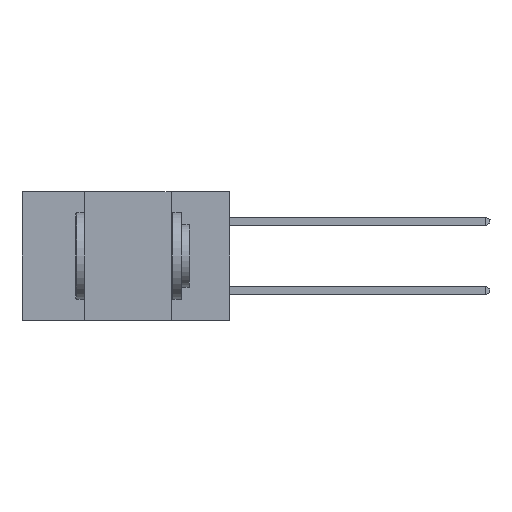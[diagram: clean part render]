
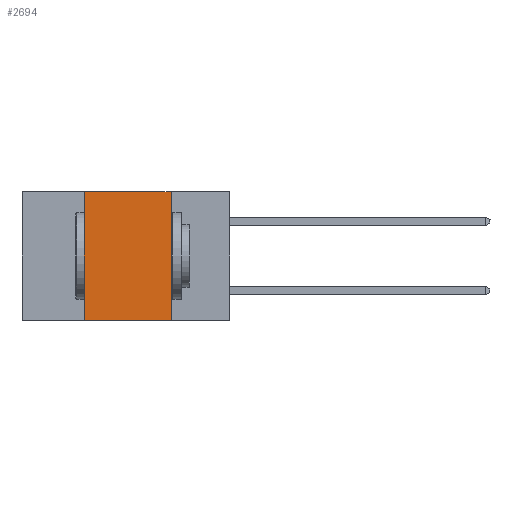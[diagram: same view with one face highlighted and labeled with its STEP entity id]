
A CAD part, left-side view. The second image highlights one B-rep face of the part: STEP entity #2694.
In plain terms, the highlighted planar face has unit normal (-1, 0, 0).
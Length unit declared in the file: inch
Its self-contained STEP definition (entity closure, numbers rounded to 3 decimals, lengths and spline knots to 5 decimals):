
#430 = PLANE ( 'NONE',  #3538 ) ;
#1069 = EDGE_CURVE ( 'NONE', #6227, #9519, #11426, .T. ) ;
#1264 = DIRECTION ( 'NONE',  ( 0., -1., 0. ) ) ;
#1434 = CARTESIAN_POINT ( 'NONE',  ( 0., 0.17, 0. ) ) ;
#1588 = ORIENTED_EDGE ( 'NONE', *, *, #3224, .F. ) ;
#1953 = CARTESIAN_POINT ( 'NONE',  ( 0., 0.42, 0. ) ) ;
#2218 = VECTOR ( 'NONE', #1264, 39.37008 ) ;
#2261 = CARTESIAN_POINT ( 'NONE',  ( 0., 0.6, 0. ) ) ;
#2622 = LINE ( 'NONE', #6323, #10069 ) ;
#2694 = ADVANCED_FACE ( 'NONE', ( #3941 ), #430, .F. ) ;
#3100 = VERTEX_POINT ( 'NONE', #10593 ) ;
#3224 = EDGE_CURVE ( 'NONE', #3100, #11199, #6571, .T. ) ;
#3456 = ORIENTED_EDGE ( 'NONE', *, *, #9744, .F. ) ;
#3538 = AXIS2_PLACEMENT_3D ( 'NONE', #2261, #11786, #7277 ) ;
#3569 = VECTOR ( 'NONE', #5542, 39.37008 ) ;
#3767 = ORIENTED_EDGE ( 'NONE', *, *, #1069, .F. ) ;
#3941 = FACE_OUTER_BOUND ( 'NONE', #8736, .T. ) ;
#4104 = LINE ( 'NONE', #7744, #2218 ) ;
#4248 = DIRECTION ( 'NONE',  ( 0., 0., 1. ) ) ;
#4286 = CARTESIAN_POINT ( 'NONE',  ( 0., 0.42, 0. ) ) ;
#4644 = CARTESIAN_POINT ( 'NONE',  ( 0., 0.17, -0.37 ) ) ;
#5542 = DIRECTION ( 'NONE',  ( 0., 0., -1. ) ) ;
#6227 = VERTEX_POINT ( 'NONE', #1434 ) ;
#6292 = VECTOR ( 'NONE', #4248, 39.37008 ) ;
#6323 = CARTESIAN_POINT ( 'NONE',  ( 0., 0.6, -0.37 ) ) ;
#6571 = LINE ( 'NONE', #4286, #6292 ) ;
#7105 = ORIENTED_EDGE ( 'NONE', *, *, #11830, .T. ) ;
#7277 = DIRECTION ( 'NONE',  ( 0., 0., -1. ) ) ;
#7744 = CARTESIAN_POINT ( 'NONE',  ( 0., 0.6, 0. ) ) ;
#8736 = EDGE_LOOP ( 'NONE', ( #3767, #3456, #1588, #7105 ) ) ;
#8795 = CARTESIAN_POINT ( 'NONE',  ( 0., 0.17, 0. ) ) ;
#9037 = DIRECTION ( 'NONE',  ( 0., -1., 0. ) ) ;
#9519 = VERTEX_POINT ( 'NONE', #4644 ) ;
#9744 = EDGE_CURVE ( 'NONE', #11199, #6227, #4104, .T. ) ;
#10069 = VECTOR ( 'NONE', #9037, 39.37008 ) ;
#10593 = CARTESIAN_POINT ( 'NONE',  ( 0., 0.42, -0.37 ) ) ;
#11199 = VERTEX_POINT ( 'NONE', #1953 ) ;
#11426 = LINE ( 'NONE', #8795, #3569 ) ;
#11786 = DIRECTION ( 'NONE',  ( 1., 0., 0. ) ) ;
#11830 = EDGE_CURVE ( 'NONE', #3100, #9519, #2622, .T. ) ;
